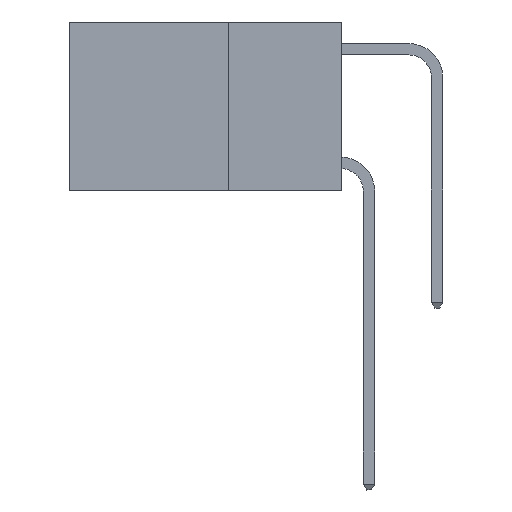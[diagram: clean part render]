
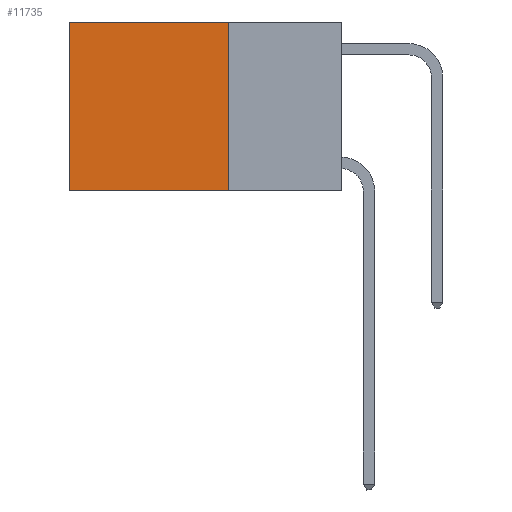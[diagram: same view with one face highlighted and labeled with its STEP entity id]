
A CAD part, left-side view. The second image highlights one B-rep face of the part: STEP entity #11735.
In plain terms, the highlighted planar face has unit normal (-1, 0, 0).
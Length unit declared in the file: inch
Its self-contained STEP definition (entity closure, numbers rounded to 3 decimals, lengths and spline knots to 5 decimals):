
#396 = VERTEX_POINT ( 'NONE', #15164 ) ;
#1042 = DIRECTION ( 'NONE',  ( 0., 1., 0. ) ) ;
#1765 = DIRECTION ( 'NONE',  ( 0., 1., 0. ) ) ;
#1802 = DIRECTION ( 'NONE',  ( 0., 0., -1. ) ) ;
#3404 = CARTESIAN_POINT ( 'NONE',  ( 0.2625, 0.25, -0.37 ) ) ;
#4026 = DIRECTION ( 'NONE',  ( 0., 0., -1. ) ) ;
#4486 = PLANE ( 'NONE',  #10931 ) ;
#4720 = EDGE_CURVE ( 'NONE', #8194, #396, #29785, .T. ) ;
#6950 = CARTESIAN_POINT ( 'NONE',  ( 0.2625, 0.6, -0.37 ) ) ;
#8114 = EDGE_CURVE ( 'NONE', #26387, #30444, #8123, .T. ) ;
#8123 = LINE ( 'NONE', #3404, #13019 ) ;
#8194 = VERTEX_POINT ( 'NONE', #25402 ) ;
#10931 = AXIS2_PLACEMENT_3D ( 'NONE', #11834, #28685, #14243 ) ;
#11087 = VECTOR ( 'NONE', #1802, 39.37008 ) ;
#11735 = ADVANCED_FACE ( 'NONE', ( #12634 ), #4486, .F. ) ;
#11834 = CARTESIAN_POINT ( 'NONE',  ( 0.2625, 0.25, 0. ) ) ;
#12316 = EDGE_CURVE ( 'NONE', #396, #30444, #16729, .T. ) ;
#12634 = FACE_OUTER_BOUND ( 'NONE', #18583, .T. ) ;
#13019 = VECTOR ( 'NONE', #1042, 39.37008 ) ;
#13678 = CARTESIAN_POINT ( 'NONE',  ( 0.2625, 0.25, 0. ) ) ;
#14186 = ORIENTED_EDGE ( 'NONE', *, *, #12316, .T. ) ;
#14243 = DIRECTION ( 'NONE',  ( 0., 0., -1. ) ) ;
#14629 = VECTOR ( 'NONE', #4026, 39.37008 ) ;
#15164 = CARTESIAN_POINT ( 'NONE',  ( 0.2625, 0.6, 0. ) ) ;
#16315 = CARTESIAN_POINT ( 'NONE',  ( 0.2625, 0.6, 0. ) ) ;
#16729 = LINE ( 'NONE', #16315, #11087 ) ;
#16967 = VECTOR ( 'NONE', #1765, 39.37008 ) ;
#17355 = CARTESIAN_POINT ( 'NONE',  ( 0.2625, 0.25, -0.37 ) ) ;
#18583 = EDGE_LOOP ( 'NONE', ( #14186, #29868, #23475, #26788 ) ) ;
#20300 = LINE ( 'NONE', #13678, #14629 ) ;
#23475 = ORIENTED_EDGE ( 'NONE', *, *, #30339, .F. ) ;
#25402 = CARTESIAN_POINT ( 'NONE',  ( 0.2625, 0.25, 0. ) ) ;
#26387 = VERTEX_POINT ( 'NONE', #17355 ) ;
#26788 = ORIENTED_EDGE ( 'NONE', *, *, #4720, .T. ) ;
#28685 = DIRECTION ( 'NONE',  ( 1., 0., 0. ) ) ;
#29785 = LINE ( 'NONE', #30694, #16967 ) ;
#29868 = ORIENTED_EDGE ( 'NONE', *, *, #8114, .F. ) ;
#30339 = EDGE_CURVE ( 'NONE', #8194, #26387, #20300, .T. ) ;
#30444 = VERTEX_POINT ( 'NONE', #6950 ) ;
#30694 = CARTESIAN_POINT ( 'NONE',  ( 0.2625, 0.25, 0. ) ) ;
